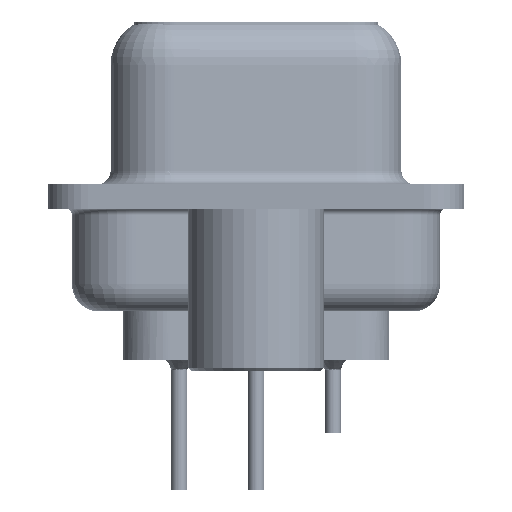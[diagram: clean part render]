
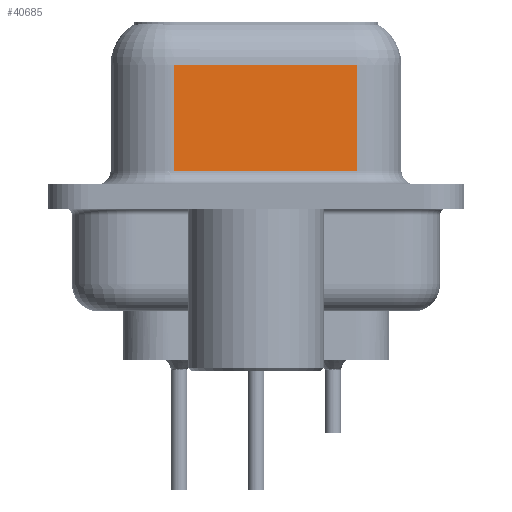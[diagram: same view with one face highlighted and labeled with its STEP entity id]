
A CAD part, left-side view. The second image highlights one B-rep face of the part: STEP entity #40685.
In plain terms, the highlighted planar face has unit normal (-0.985, -0.174, 0).
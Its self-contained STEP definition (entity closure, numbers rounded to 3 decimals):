
#635 = CARTESIAN_POINT ( 'NONE',  ( 5.621, -3.722, 6.6 ) ) ;
#1735 = DIRECTION ( 'NONE',  ( -0.174, 0.985, 0. ) ) ;
#2880 = VECTOR ( 'NONE', #1735, 1000. ) ;
#3062 = PLANE ( 'NONE',  #19361 ) ;
#3416 = EDGE_CURVE ( 'NONE', #27322, #36946, #31496, .T. ) ;
#4493 = CARTESIAN_POINT ( 'NONE',  ( 5.621, -3.722, 0.95 ) ) ;
#5530 = CARTESIAN_POINT ( 'NONE',  ( 4.43, 3.028, 6.6 ) ) ;
#7657 = VECTOR ( 'NONE', #31390, 1000. ) ;
#8051 = CARTESIAN_POINT ( 'NONE',  ( 5.621, -3.722, 4.85 ) ) ;
#12689 = DIRECTION ( 'NONE',  ( 0.174, -0.985, 0. ) ) ;
#14326 = EDGE_LOOP ( 'NONE', ( #14605, #20342, #38639, #23385 ) ) ;
#14605 = ORIENTED_EDGE ( 'NONE', *, *, #28685, .F. ) ;
#19361 = AXIS2_PLACEMENT_3D ( 'NONE', #19791, #39984, #29357 ) ;
#19791 = CARTESIAN_POINT ( 'NONE',  ( 5.621, -3.722, 6.6 ) ) ;
#20189 = DIRECTION ( 'NONE',  ( 0., 0., -1. ) ) ;
#20342 = ORIENTED_EDGE ( 'NONE', *, *, #3416, .T. ) ;
#20880 = CARTESIAN_POINT ( 'NONE',  ( 4.43, 3.028, 0.95 ) ) ;
#22279 = LINE ( 'NONE', #5530, #7657 ) ;
#23267 = EDGE_CURVE ( 'NONE', #36946, #27072, #22279, .T. ) ;
#23385 = ORIENTED_EDGE ( 'NONE', *, *, #33066, .T. ) ;
#23888 = VECTOR ( 'NONE', #20189, 1000. ) ;
#26406 = CARTESIAN_POINT ( 'NONE',  ( 5.621, -3.722, 0.95 ) ) ;
#27072 = VERTEX_POINT ( 'NONE', #20880 ) ;
#27322 = VERTEX_POINT ( 'NONE', #35804 ) ;
#28685 = EDGE_CURVE ( 'NONE', #27322, #40137, #37081, .T. ) ;
#28800 = CARTESIAN_POINT ( 'NONE',  ( 4.43, 3.028, 4.85 ) ) ;
#29357 = DIRECTION ( 'NONE',  ( -0.174, 0.985, 0. ) ) ;
#31390 = DIRECTION ( 'NONE',  ( 0., 0., -1. ) ) ;
#31496 = LINE ( 'NONE', #8051, #2880 ) ;
#33066 = EDGE_CURVE ( 'NONE', #27072, #40137, #36329, .T. ) ;
#35804 = CARTESIAN_POINT ( 'NONE',  ( 5.621, -3.722, 4.85 ) ) ;
#36329 = LINE ( 'NONE', #26406, #39341 ) ;
#36946 = VERTEX_POINT ( 'NONE', #28800 ) ;
#37081 = LINE ( 'NONE', #635, #23888 ) ;
#38639 = ORIENTED_EDGE ( 'NONE', *, *, #23267, .T. ) ;
#39341 = VECTOR ( 'NONE', #12689, 1000. ) ;
#39984 = DIRECTION ( 'NONE',  ( 0.985, 0.174, 0. ) ) ;
#40137 = VERTEX_POINT ( 'NONE', #4493 ) ;
#40685 = ADVANCED_FACE ( 'NONE', ( #42847 ), #3062, .F. ) ;
#42847 = FACE_OUTER_BOUND ( 'NONE', #14326, .T. ) ;
